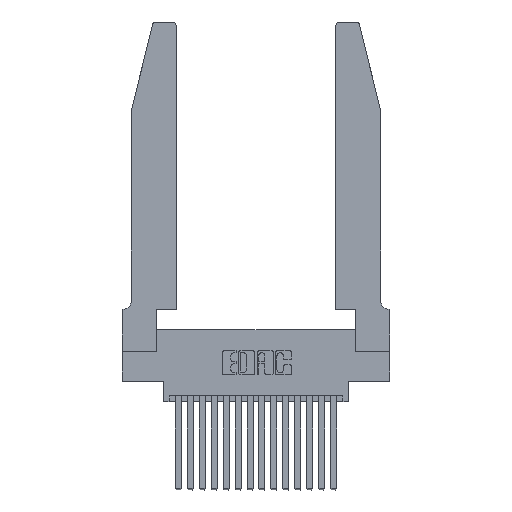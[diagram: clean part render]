
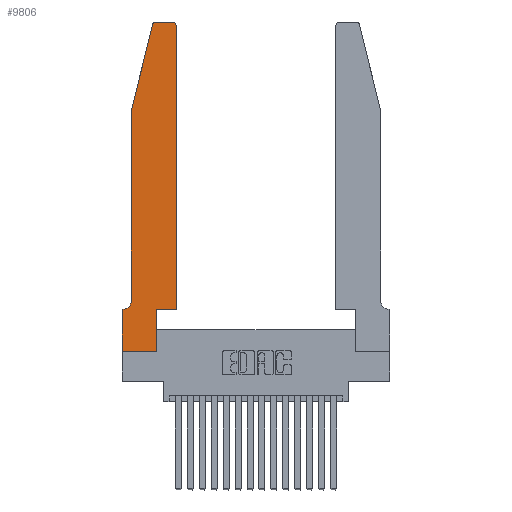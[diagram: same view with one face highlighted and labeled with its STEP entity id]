
A CAD part, top view. The second image highlights one B-rep face of the part: STEP entity #9806.
In plain terms, the highlighted planar face has unit normal (0, 0, 1).
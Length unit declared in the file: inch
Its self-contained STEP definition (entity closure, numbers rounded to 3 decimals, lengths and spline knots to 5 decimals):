
#111 = LINE ( 'NONE', #12423, #11476 ) ;
#130 = CARTESIAN_POINT ( 'NONE',  ( 0., 0., 0.37 ) ) ;
#149 = DIRECTION ( 'NONE',  ( -0.239, -0.971, 0. ) ) ;
#236 = CARTESIAN_POINT ( 'NONE',  ( 0.0055, 0.35, 0.37 ) ) ;
#962 = EDGE_CURVE ( 'NONE', #18384, #18544, #19120, .T. ) ;
#969 = CARTESIAN_POINT ( 'NONE',  ( 0.0055, 0.42, 0.37 ) ) ;
#1018 = CARTESIAN_POINT ( 'NONE',  ( 0.284, 2.72, 0.37 ) ) ;
#1412 = ORIENTED_EDGE ( 'NONE', *, *, #5850, .T. ) ;
#2494 = EDGE_CURVE ( 'NONE', #18544, #17128, #3223, .T. ) ;
#2541 = DIRECTION ( 'NONE',  ( -1., 0., 0. ) ) ;
#2579 = ORIENTED_EDGE ( 'NONE', *, *, #2494, .T. ) ;
#2598 = DIRECTION ( 'NONE',  ( 1., 0., 0. ) ) ;
#2930 = DIRECTION ( 'NONE',  ( 0., -1., 0. ) ) ;
#3015 = CARTESIAN_POINT ( 'NONE',  ( 0.2865, 0., 0.37 ) ) ;
#3199 = AXIS2_PLACEMENT_3D ( 'NONE', #969, #11742, #2541 ) ;
#3216 = CIRCLE ( 'NONE', #6631, 0.03 ) ;
#3223 = LINE ( 'NONE', #17691, #10930 ) ;
#3310 = EDGE_LOOP ( 'NONE', ( #11898, #8263, #5347, #2579, #5635, #17223, #9709, #1412, #16803, #10937, #3720, #13289 ) ) ;
#3546 = DIRECTION ( 'NONE',  ( 0., 1., 0. ) ) ;
#3720 = ORIENTED_EDGE ( 'NONE', *, *, #8416, .T. ) ;
#3847 = VERTEX_POINT ( 'NONE', #3015 ) ;
#3888 = DIRECTION ( 'NONE',  ( 0., 0., 1. ) ) ;
#3977 = CARTESIAN_POINT ( 'NONE',  ( 0.4505, 2.72, 0.37 ) ) ;
#4132 = CARTESIAN_POINT ( 'NONE',  ( 0.0755, 0.42, 0.37 ) ) ;
#4180 = VERTEX_POINT ( 'NONE', #8875 ) ;
#4619 = CARTESIAN_POINT ( 'NONE',  ( 0.4205, 2.75, 0.37 ) ) ;
#4760 = PLANE ( 'NONE',  #5093 ) ;
#5093 = AXIS2_PLACEMENT_3D ( 'NONE', #9340, #15160, #6336 ) ;
#5269 = EDGE_CURVE ( 'NONE', #4180, #12509, #8029, .T. ) ;
#5347 = ORIENTED_EDGE ( 'NONE', *, *, #962, .T. ) ;
#5635 = ORIENTED_EDGE ( 'NONE', *, *, #17117, .T. ) ;
#5819 = DIRECTION ( 'NONE',  ( 1., 0., 0. ) ) ;
#5850 = EDGE_CURVE ( 'NONE', #11411, #3847, #10099, .T. ) ;
#6336 = DIRECTION ( 'NONE',  ( 1., 0., 0. ) ) ;
#6631 = AXIS2_PLACEMENT_3D ( 'NONE', #1018, #11793, #2598 ) ;
#7526 = VECTOR ( 'NONE', #12591, 39.37008 ) ;
#7562 = LINE ( 'NONE', #14064, #11096 ) ;
#7884 = LINE ( 'NONE', #17397, #15178 ) ;
#7991 = CARTESIAN_POINT ( 'NONE',  ( 0.0755, 2., 0.37 ) ) ;
#8029 = LINE ( 'NONE', #18295, #7526 ) ;
#8263 = ORIENTED_EDGE ( 'NONE', *, *, #8434, .T. ) ;
#8416 = EDGE_CURVE ( 'NONE', #12509, #17664, #7884, .T. ) ;
#8434 = EDGE_CURVE ( 'NONE', #18620, #18384, #3216, .T. ) ;
#8875 = CARTESIAN_POINT ( 'NONE',  ( 0.2865, 0.35, 0.37 ) ) ;
#8912 = LINE ( 'NONE', #11183, #16173 ) ;
#8994 = DIRECTION ( 'NONE',  ( 0., -1., 0. ) ) ;
#9340 = CARTESIAN_POINT ( 'NONE',  ( 0., 0.35, 0.37 ) ) ;
#9709 = ORIENTED_EDGE ( 'NONE', *, *, #11943, .T. ) ;
#9741 = VERTEX_POINT ( 'NONE', #4619 ) ;
#9806 = ADVANCED_FACE ( 'NONE', ( #11780 ), #4760, .T. ) ;
#10099 = LINE ( 'NONE', #16145, #13978 ) ;
#10843 = VERTEX_POINT ( 'NONE', #236 ) ;
#10930 = VECTOR ( 'NONE', #8994, 39.37008 ) ;
#10937 = ORIENTED_EDGE ( 'NONE', *, *, #5269, .T. ) ;
#11096 = VECTOR ( 'NONE', #15495, 39.37008 ) ;
#11183 = CARTESIAN_POINT ( 'NONE',  ( 0.2865, 0.35, 0.37 ) ) ;
#11316 = LINE ( 'NONE', #13381, #18979 ) ;
#11411 = VERTEX_POINT ( 'NONE', #130 ) ;
#11476 = VECTOR ( 'NONE', #2930, 39.37008 ) ;
#11603 = DIRECTION ( 'NONE',  ( 0., 1., 0. ) ) ;
#11742 = DIRECTION ( 'NONE',  ( 0., 0., -1. ) ) ;
#11780 = FACE_OUTER_BOUND ( 'NONE', #3310, .T. ) ;
#11793 = DIRECTION ( 'NONE',  ( 0., 0., 1. ) ) ;
#11898 = ORIENTED_EDGE ( 'NONE', *, *, #14557, .T. ) ;
#11943 = EDGE_CURVE ( 'NONE', #16926, #11411, #111, .T. ) ;
#12423 = CARTESIAN_POINT ( 'NONE',  ( 0., 0., 0.37 ) ) ;
#12490 = CIRCLE ( 'NONE', #13092, 0.03 ) ;
#12509 = VERTEX_POINT ( 'NONE', #17864 ) ;
#12591 = DIRECTION ( 'NONE',  ( 1., 0., 0. ) ) ;
#12830 = CARTESIAN_POINT ( 'NONE',  ( 0., 0.35, 0.37 ) ) ;
#12969 = CARTESIAN_POINT ( 'NONE',  ( 0.4205, 2.72, 0.37 ) ) ;
#13092 = AXIS2_PLACEMENT_3D ( 'NONE', #12969, #3888, #14383 ) ;
#13289 = ORIENTED_EDGE ( 'NONE', *, *, #14088, .T. ) ;
#13381 = CARTESIAN_POINT ( 'NONE',  ( 0.0755, 0.35, 0.37 ) ) ;
#13978 = VECTOR ( 'NONE', #5819, 39.37008 ) ;
#14064 = CARTESIAN_POINT ( 'NONE',  ( 0.2605, 2.75, 0.37 ) ) ;
#14088 = EDGE_CURVE ( 'NONE', #17664, #9741, #12490, .T. ) ;
#14383 = DIRECTION ( 'NONE',  ( 1., 0., 0. ) ) ;
#14557 = EDGE_CURVE ( 'NONE', #9741, #18620, #7562, .T. ) ;
#14779 = EDGE_CURVE ( 'NONE', #10843, #16926, #11316, .T. ) ;
#15160 = DIRECTION ( 'NONE',  ( 0., 0., 1. ) ) ;
#15178 = VECTOR ( 'NONE', #11603, 39.37008 ) ;
#15245 = VECTOR ( 'NONE', #149, 39.37008 ) ;
#15495 = DIRECTION ( 'NONE',  ( -1., 0., 0. ) ) ;
#15879 = CARTESIAN_POINT ( 'NONE',  ( 0.25487, 2.72718, 0.37 ) ) ;
#16145 = CARTESIAN_POINT ( 'NONE',  ( 0., 0., 0.37 ) ) ;
#16173 = VECTOR ( 'NONE', #3546, 39.37008 ) ;
#16390 = CIRCLE ( 'NONE', #3199, 0.07 ) ;
#16803 = ORIENTED_EDGE ( 'NONE', *, *, #16850, .T. ) ;
#16850 = EDGE_CURVE ( 'NONE', #3847, #4180, #8912, .T. ) ;
#16926 = VERTEX_POINT ( 'NONE', #12830 ) ;
#17117 = EDGE_CURVE ( 'NONE', #17128, #10843, #16390, .T. ) ;
#17128 = VERTEX_POINT ( 'NONE', #4132 ) ;
#17223 = ORIENTED_EDGE ( 'NONE', *, *, #14779, .T. ) ;
#17397 = CARTESIAN_POINT ( 'NONE',  ( 0.4505, 0.35, 0.37 ) ) ;
#17664 = VERTEX_POINT ( 'NONE', #3977 ) ;
#17691 = CARTESIAN_POINT ( 'NONE',  ( 0.0755, 2., 0.37 ) ) ;
#17864 = CARTESIAN_POINT ( 'NONE',  ( 0.4505, 0.35, 0.37 ) ) ;
#18295 = CARTESIAN_POINT ( 'NONE',  ( 0.4505, 0.35, 0.37 ) ) ;
#18361 = CARTESIAN_POINT ( 'NONE',  ( 0.284, 2.75, 0.37 ) ) ;
#18384 = VERTEX_POINT ( 'NONE', #15879 ) ;
#18544 = VERTEX_POINT ( 'NONE', #7991 ) ;
#18620 = VERTEX_POINT ( 'NONE', #18361 ) ;
#18914 = CARTESIAN_POINT ( 'NONE',  ( 0.0755, 2., 0.37 ) ) ;
#18979 = VECTOR ( 'NONE', #19119, 39.37008 ) ;
#19119 = DIRECTION ( 'NONE',  ( -1., 0., 0. ) ) ;
#19120 = LINE ( 'NONE', #18914, #15245 ) ;
